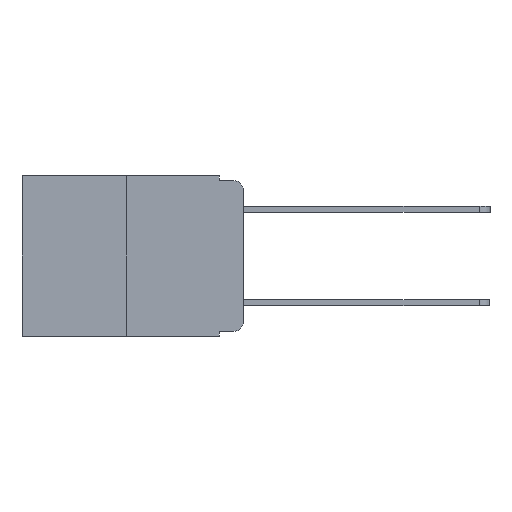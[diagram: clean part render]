
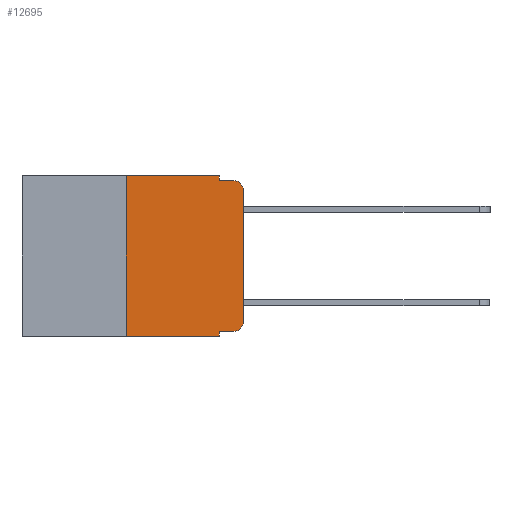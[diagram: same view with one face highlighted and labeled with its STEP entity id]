
A CAD part, left-side view. The second image highlights one B-rep face of the part: STEP entity #12695.
In plain terms, the highlighted planar face has unit normal (-1, 0, 0).
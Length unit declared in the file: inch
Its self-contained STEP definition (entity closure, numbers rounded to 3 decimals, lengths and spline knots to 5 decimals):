
#68 = CARTESIAN_POINT ( 'NONE',  ( 0., 0.051, -0.01 ) ) ;
#348 = VERTEX_POINT ( 'NONE', #12101 ) ;
#417 = EDGE_CURVE ( 'NONE', #20270, #348, #9458, .T. ) ;
#598 = VECTOR ( 'NONE', #17081, 39.37008 ) ;
#781 = ORIENTED_EDGE ( 'NONE', *, *, #5662, .F. ) ;
#854 = DIRECTION ( 'NONE',  ( -1., 0., 0. ) ) ;
#1147 = PLANE ( 'NONE',  #20201 ) ;
#1855 = ORIENTED_EDGE ( 'NONE', *, *, #3103, .F. ) ;
#1993 = CARTESIAN_POINT ( 'NONE',  ( 0., 0.051, 0. ) ) ;
#2750 = EDGE_CURVE ( 'NONE', #18814, #17697, #5024, .T. ) ;
#2885 = CARTESIAN_POINT ( 'NONE',  ( 0., 0.051, 0. ) ) ;
#2888 = LINE ( 'NONE', #2885, #12881 ) ;
#2930 = ORIENTED_EDGE ( 'NONE', *, *, #417, .F. ) ;
#2958 = ORIENTED_EDGE ( 'NONE', *, *, #8964, .T. ) ;
#3037 = CARTESIAN_POINT ( 'NONE',  ( 0., 0.02, -0.333 ) ) ;
#3103 = EDGE_CURVE ( 'NONE', #14685, #19172, #2888, .T. ) ;
#3472 = DIRECTION ( 'NONE',  ( 0., -1., 0. ) ) ;
#3551 = ORIENTED_EDGE ( 'NONE', *, *, #7365, .T. ) ;
#4550 = CARTESIAN_POINT ( 'NONE',  ( 0., 0.02, -0.03 ) ) ;
#4740 = ORIENTED_EDGE ( 'NONE', *, *, #2750, .T. ) ;
#5024 = CIRCLE ( 'NONE', #16378, 0.02 ) ;
#5483 = VECTOR ( 'NONE', #17047, 39.37008 ) ;
#5662 = EDGE_CURVE ( 'NONE', #19172, #15220, #6633, .T. ) ;
#5791 = LINE ( 'NONE', #1993, #598 ) ;
#6426 = DIRECTION ( 'NONE',  ( 0., 0., -1. ) ) ;
#6523 = VECTOR ( 'NONE', #12034, 39.37008 ) ;
#6633 = LINE ( 'NONE', #68, #5483 ) ;
#6972 = CARTESIAN_POINT ( 'NONE',  ( 0., 0.473, 0. ) ) ;
#7156 = LINE ( 'NONE', #20424, #11487 ) ;
#7365 = EDGE_CURVE ( 'NONE', #9151, #18814, #21946, .T. ) ;
#7638 = AXIS2_PLACEMENT_3D ( 'NONE', #4550, #17624, #6426 ) ;
#7723 = VERTEX_POINT ( 'NONE', #13846 ) ;
#7749 = EDGE_CURVE ( 'NONE', #348, #14685, #11460, .T. ) ;
#8513 = ORIENTED_EDGE ( 'NONE', *, *, #7749, .F. ) ;
#8629 = DIRECTION ( 'NONE',  ( 0., 0., 1. ) ) ;
#8634 = FACE_OUTER_BOUND ( 'NONE', #13007, .T. ) ;
#8964 = EDGE_CURVE ( 'NONE', #20270, #10378, #9669, .T. ) ;
#9151 = VERTEX_POINT ( 'NONE', #19856 ) ;
#9458 = LINE ( 'NONE', #23883, #14478 ) ;
#9669 = LINE ( 'NONE', #15531, #14697 ) ;
#10378 = VERTEX_POINT ( 'NONE', #22443 ) ;
#10668 = DIRECTION ( 'NONE',  ( 0., 0., -1. ) ) ;
#11460 = LINE ( 'NONE', #15828, #6523 ) ;
#11487 = VECTOR ( 'NONE', #22262, 39.37008 ) ;
#11660 = CARTESIAN_POINT ( 'NONE',  ( 0., 0.02, -0.01 ) ) ;
#11814 = DIRECTION ( 'NONE',  ( 0., -1., 0. ) ) ;
#12034 = DIRECTION ( 'NONE',  ( 0., -1., 0. ) ) ;
#12092 = VECTOR ( 'NONE', #3472, 39.37008 ) ;
#12101 = CARTESIAN_POINT ( 'NONE',  ( 0., 0.25, 0. ) ) ;
#12695 = ADVANCED_FACE ( 'NONE', ( #8634 ), #1147, .F. ) ;
#12803 = CARTESIAN_POINT ( 'NONE',  ( 0., 0.051, -0.333 ) ) ;
#12881 = VECTOR ( 'NONE', #20189, 39.37008 ) ;
#13007 = EDGE_LOOP ( 'NONE', ( #15256, #17138, #781, #1855, #8513, #2930, #2958, #20777, #3551, #4740 ) ) ;
#13846 = CARTESIAN_POINT ( 'NONE',  ( 0., 0., -0.03 ) ) ;
#13944 = EDGE_CURVE ( 'NONE', #17697, #7723, #7156, .T. ) ;
#14109 = CARTESIAN_POINT ( 'NONE',  ( 0., 0., -0.313 ) ) ;
#14121 = DIRECTION ( 'NONE',  ( 0., 0., -1. ) ) ;
#14478 = VECTOR ( 'NONE', #8629, 39.37008 ) ;
#14685 = VERTEX_POINT ( 'NONE', #19105 ) ;
#14697 = VECTOR ( 'NONE', #11814, 39.37008 ) ;
#15220 = VERTEX_POINT ( 'NONE', #11660 ) ;
#15256 = ORIENTED_EDGE ( 'NONE', *, *, #13944, .T. ) ;
#15531 = CARTESIAN_POINT ( 'NONE',  ( 0., 0.473, -0.343 ) ) ;
#15828 = CARTESIAN_POINT ( 'NONE',  ( 0., 0.473, 0. ) ) ;
#16378 = AXIS2_PLACEMENT_3D ( 'NONE', #16736, #854, #14121 ) ;
#16736 = CARTESIAN_POINT ( 'NONE',  ( 0., 0.02, -0.313 ) ) ;
#17047 = DIRECTION ( 'NONE',  ( 0., -1., 0. ) ) ;
#17081 = DIRECTION ( 'NONE',  ( 0., 0., -1. ) ) ;
#17138 = ORIENTED_EDGE ( 'NONE', *, *, #18169, .T. ) ;
#17397 = EDGE_CURVE ( 'NONE', #9151, #10378, #5791, .T. ) ;
#17624 = DIRECTION ( 'NONE',  ( -1., 0., 0. ) ) ;
#17697 = VERTEX_POINT ( 'NONE', #14109 ) ;
#18169 = EDGE_CURVE ( 'NONE', #7723, #15220, #23441, .T. ) ;
#18814 = VERTEX_POINT ( 'NONE', #3037 ) ;
#19105 = CARTESIAN_POINT ( 'NONE',  ( 0., 0.051, 0. ) ) ;
#19172 = VERTEX_POINT ( 'NONE', #22708 ) ;
#19856 = CARTESIAN_POINT ( 'NONE',  ( 0., 0.051, -0.333 ) ) ;
#20189 = DIRECTION ( 'NONE',  ( 0., 0., -1. ) ) ;
#20201 = AXIS2_PLACEMENT_3D ( 'NONE', #6972, #21807, #10668 ) ;
#20270 = VERTEX_POINT ( 'NONE', #21918 ) ;
#20424 = CARTESIAN_POINT ( 'NONE',  ( 0., 0., 0. ) ) ;
#20777 = ORIENTED_EDGE ( 'NONE', *, *, #17397, .F. ) ;
#21807 = DIRECTION ( 'NONE',  ( 1., 0., 0. ) ) ;
#21918 = CARTESIAN_POINT ( 'NONE',  ( 0., 0.25, -0.343 ) ) ;
#21946 = LINE ( 'NONE', #12803, #12092 ) ;
#22262 = DIRECTION ( 'NONE',  ( 0., 0., 1. ) ) ;
#22443 = CARTESIAN_POINT ( 'NONE',  ( 0., 0.051, -0.343 ) ) ;
#22708 = CARTESIAN_POINT ( 'NONE',  ( 0., 0.051, -0.01 ) ) ;
#23441 = CIRCLE ( 'NONE', #7638, 0.02 ) ;
#23883 = CARTESIAN_POINT ( 'NONE',  ( 0., 0.25, 0. ) ) ;
